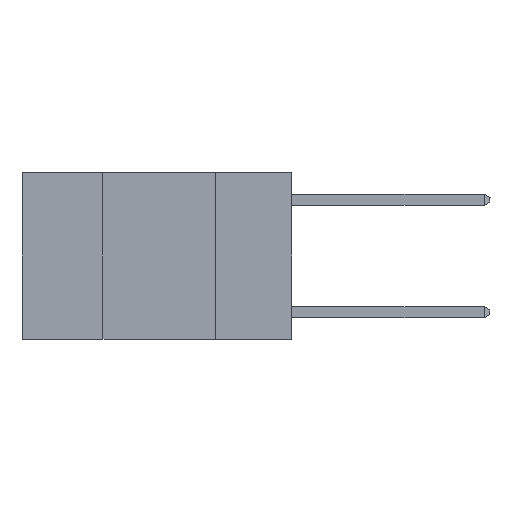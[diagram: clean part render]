
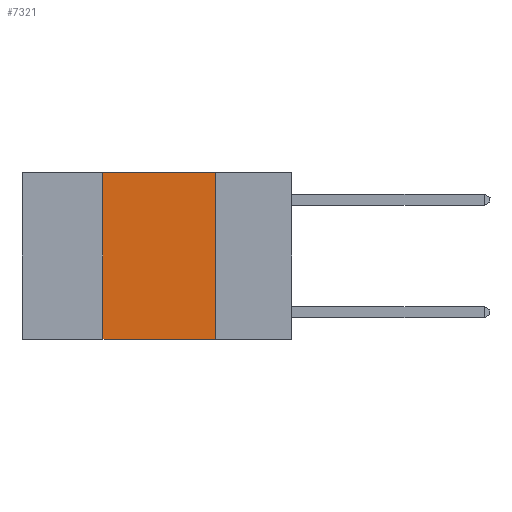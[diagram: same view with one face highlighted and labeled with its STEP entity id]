
A CAD part, left-side view. The second image highlights one B-rep face of the part: STEP entity #7321.
In plain terms, the highlighted planar face has unit normal (-1, 0, 0).
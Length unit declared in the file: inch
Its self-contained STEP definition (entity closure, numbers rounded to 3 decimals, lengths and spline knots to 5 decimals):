
#170 = EDGE_CURVE ( 'NONE', #3620, #2231, #3221, .T. ) ;
#1672 = CARTESIAN_POINT ( 'NONE',  ( 0., 0.17, -0.37 ) ) ;
#1673 = PLANE ( 'NONE',  #9375 ) ;
#1710 = CARTESIAN_POINT ( 'NONE',  ( 0., 0.6, 0. ) ) ;
#2231 = VERTEX_POINT ( 'NONE', #1672 ) ;
#3221 = LINE ( 'NONE', #6995, #4855 ) ;
#3620 = VERTEX_POINT ( 'NONE', #5838 ) ;
#3702 = ORIENTED_EDGE ( 'NONE', *, *, #170, .T. ) ;
#4164 = ORIENTED_EDGE ( 'NONE', *, *, #5120, .F. ) ;
#4353 = CARTESIAN_POINT ( 'NONE',  ( 0., 0.42, 0. ) ) ;
#4466 = DIRECTION ( 'NONE',  ( 1., 0., 0. ) ) ;
#4590 = DIRECTION ( 'NONE',  ( 0., 0., -1. ) ) ;
#4650 = EDGE_CURVE ( 'NONE', #6741, #11903, #10365, .T. ) ;
#4855 = VECTOR ( 'NONE', #5975, 39.37008 ) ;
#4897 = ORIENTED_EDGE ( 'NONE', *, *, #6651, .F. ) ;
#5120 = EDGE_CURVE ( 'NONE', #3620, #6741, #9539, .T. ) ;
#5191 = VECTOR ( 'NONE', #9668, 39.37008 ) ;
#5528 = CARTESIAN_POINT ( 'NONE',  ( 0., 0.6, 0. ) ) ;
#5563 = DIRECTION ( 'NONE',  ( 0., -1., 0. ) ) ;
#5838 = CARTESIAN_POINT ( 'NONE',  ( 0., 0.42, -0.37 ) ) ;
#5975 = DIRECTION ( 'NONE',  ( 0., -1., 0. ) ) ;
#6651 = EDGE_CURVE ( 'NONE', #11903, #2231, #11856, .T. ) ;
#6741 = VERTEX_POINT ( 'NONE', #4353 ) ;
#6995 = CARTESIAN_POINT ( 'NONE',  ( 0., 0.6, -0.37 ) ) ;
#7052 = ORIENTED_EDGE ( 'NONE', *, *, #4650, .F. ) ;
#7321 = ADVANCED_FACE ( 'NONE', ( #12204 ), #1673, .F. ) ;
#7787 = EDGE_LOOP ( 'NONE', ( #4897, #7052, #4164, #3702 ) ) ;
#9375 = AXIS2_PLACEMENT_3D ( 'NONE', #5528, #4466, #4590 ) ;
#9408 = VECTOR ( 'NONE', #5563, 39.37008 ) ;
#9539 = LINE ( 'NONE', #10467, #5191 ) ;
#9668 = DIRECTION ( 'NONE',  ( 0., 0., 1. ) ) ;
#9968 = DIRECTION ( 'NONE',  ( 0., 0., -1. ) ) ;
#10365 = LINE ( 'NONE', #1710, #9408 ) ;
#10467 = CARTESIAN_POINT ( 'NONE',  ( 0., 0.42, 0. ) ) ;
#10545 = CARTESIAN_POINT ( 'NONE',  ( 0., 0.17, 0. ) ) ;
#11021 = CARTESIAN_POINT ( 'NONE',  ( 0., 0.17, 0. ) ) ;
#11856 = LINE ( 'NONE', #11021, #12043 ) ;
#11903 = VERTEX_POINT ( 'NONE', #10545 ) ;
#12043 = VECTOR ( 'NONE', #9968, 39.37008 ) ;
#12204 = FACE_OUTER_BOUND ( 'NONE', #7787, .T. ) ;
